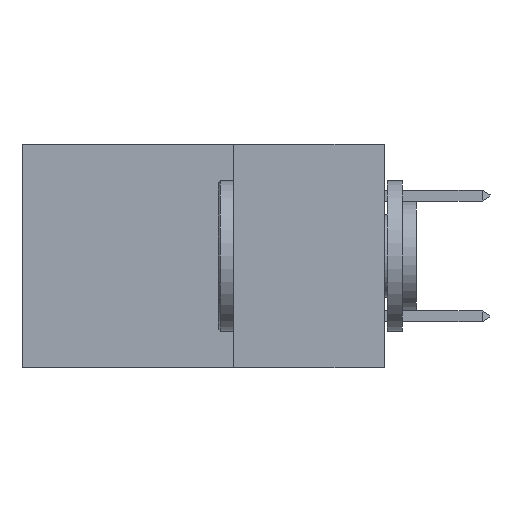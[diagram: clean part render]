
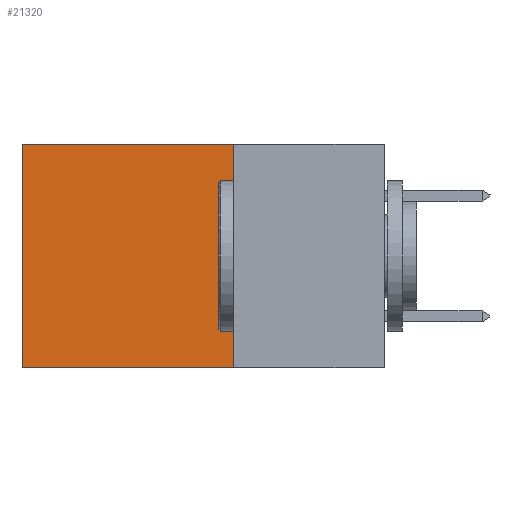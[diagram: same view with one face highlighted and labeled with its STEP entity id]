
A CAD part, left-side view. The second image highlights one B-rep face of the part: STEP entity #21320.
In plain terms, the highlighted planar face has unit normal (-1, 0, 0).
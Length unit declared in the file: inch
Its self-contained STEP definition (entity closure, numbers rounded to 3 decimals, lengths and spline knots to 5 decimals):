
#1074 = EDGE_CURVE ( 'NONE', #16392, #1427, #22570, .T. ) ;
#1427 = VERTEX_POINT ( 'NONE', #35334 ) ;
#3896 = PLANE ( 'NONE',  #19854 ) ;
#4639 = LINE ( 'NONE', #40073, #20837 ) ;
#4933 = VECTOR ( 'NONE', #31706, 39.37008 ) ;
#5571 = CARTESIAN_POINT ( 'NONE',  ( 0.2875, 0.25, 0. ) ) ;
#6075 = CARTESIAN_POINT ( 'NONE',  ( 0.2875, 0.25, -0.37 ) ) ;
#7154 = DIRECTION ( 'NONE',  ( 0., 0., -1. ) ) ;
#7296 = CARTESIAN_POINT ( 'NONE',  ( 0.2875, 0.6, 0. ) ) ;
#7306 = DIRECTION ( 'NONE',  ( 0., 0., -1. ) ) ;
#8828 = DIRECTION ( 'NONE',  ( 0., 0., -1. ) ) ;
#10419 = EDGE_CURVE ( 'NONE', #29241, #29182, #14486, .T. ) ;
#13089 = ORIENTED_EDGE ( 'NONE', *, *, #23818, .F. ) ;
#13569 = LINE ( 'NONE', #6075, #4933 ) ;
#14486 = LINE ( 'NONE', #5571, #38896 ) ;
#16392 = VERTEX_POINT ( 'NONE', #35092 ) ;
#16829 = CARTESIAN_POINT ( 'NONE',  ( 0.2875, 0.25, 0. ) ) ;
#16874 = ORIENTED_EDGE ( 'NONE', *, *, #30940, .T. ) ;
#17038 = VECTOR ( 'NONE', #7306, 39.37008 ) ;
#17721 = CARTESIAN_POINT ( 'NONE',  ( 0.2875, 0.25, 0. ) ) ;
#17850 = DIRECTION ( 'NONE',  ( 0., 1., 0. ) ) ;
#19854 = AXIS2_PLACEMENT_3D ( 'NONE', #16829, #26494, #7154 ) ;
#20837 = VECTOR ( 'NONE', #17850, 39.37008 ) ;
#21320 = ADVANCED_FACE ( 'NONE', ( #31407 ), #3896, .F. ) ;
#22570 = LINE ( 'NONE', #7296, #17038 ) ;
#23818 = EDGE_CURVE ( 'NONE', #29182, #1427, #13569, .T. ) ;
#26494 = DIRECTION ( 'NONE',  ( 1., 0., 0. ) ) ;
#29182 = VERTEX_POINT ( 'NONE', #30092 ) ;
#29241 = VERTEX_POINT ( 'NONE', #17721 ) ;
#29515 = ORIENTED_EDGE ( 'NONE', *, *, #1074, .T. ) ;
#30092 = CARTESIAN_POINT ( 'NONE',  ( 0.2875, 0.25, -0.37 ) ) ;
#30940 = EDGE_CURVE ( 'NONE', #29241, #16392, #4639, .T. ) ;
#31407 = FACE_OUTER_BOUND ( 'NONE', #33398, .T. ) ;
#31706 = DIRECTION ( 'NONE',  ( 0., 1., 0. ) ) ;
#33398 = EDGE_LOOP ( 'NONE', ( #29515, #13089, #33571, #16874 ) ) ;
#33571 = ORIENTED_EDGE ( 'NONE', *, *, #10419, .F. ) ;
#35092 = CARTESIAN_POINT ( 'NONE',  ( 0.2875, 0.6, 0. ) ) ;
#35334 = CARTESIAN_POINT ( 'NONE',  ( 0.2875, 0.6, -0.37 ) ) ;
#38896 = VECTOR ( 'NONE', #8828, 39.37008 ) ;
#40073 = CARTESIAN_POINT ( 'NONE',  ( 0.2875, 0.25, 0. ) ) ;
